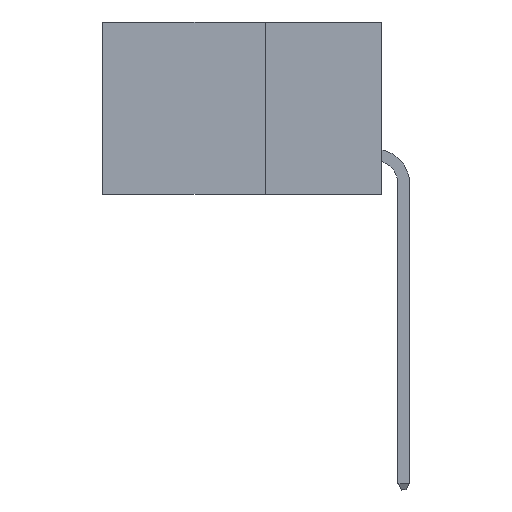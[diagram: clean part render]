
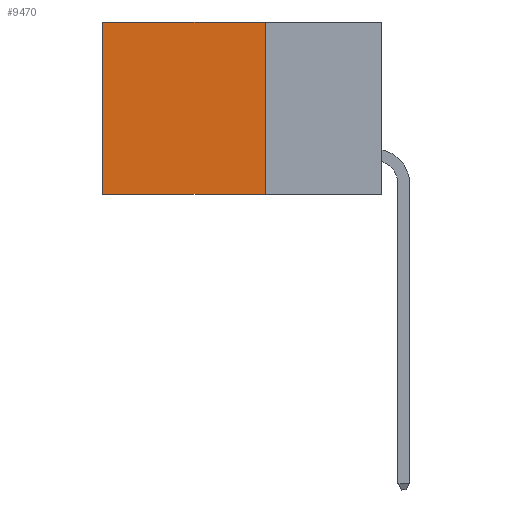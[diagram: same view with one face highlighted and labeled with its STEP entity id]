
A CAD part, left-side view. The second image highlights one B-rep face of the part: STEP entity #9470.
In plain terms, the highlighted planar face has unit normal (-1, 0, 0).
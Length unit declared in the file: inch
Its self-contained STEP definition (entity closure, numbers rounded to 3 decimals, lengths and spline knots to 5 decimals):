
#390 = LINE ( 'NONE', #29003, #17662 ) ;
#4487 = LINE ( 'NONE', #10090, #17136 ) ;
#4966 = VERTEX_POINT ( 'NONE', #17855 ) ;
#5613 = VERTEX_POINT ( 'NONE', #17283 ) ;
#7148 = EDGE_LOOP ( 'NONE', ( #9092, #29058, #9998, #28277 ) ) ;
#8031 = VECTOR ( 'NONE', #18844, 39.37008 ) ;
#8663 = DIRECTION ( 'NONE',  ( 0., 1., 0. ) ) ;
#9092 = ORIENTED_EDGE ( 'NONE', *, *, #27986, .T. ) ;
#9470 = ADVANCED_FACE ( 'NONE', ( #22668 ), #28530, .F. ) ;
#9898 = VECTOR ( 'NONE', #23428, 39.37008 ) ;
#9998 = ORIENTED_EDGE ( 'NONE', *, *, #25482, .F. ) ;
#10090 = CARTESIAN_POINT ( 'NONE',  ( 0.2875, 0.6, 0. ) ) ;
#10237 = VERTEX_POINT ( 'NONE', #28568 ) ;
#12188 = EDGE_CURVE ( 'NONE', #10237, #5613, #390, .T. ) ;
#12823 = DIRECTION ( 'NONE',  ( 1., 0., 0. ) ) ;
#13265 = LINE ( 'NONE', #14539, #8031 ) ;
#13345 = LINE ( 'NONE', #18789, #9898 ) ;
#14539 = CARTESIAN_POINT ( 'NONE',  ( 0.2875, 0.25, 0. ) ) ;
#15705 = AXIS2_PLACEMENT_3D ( 'NONE', #19302, #12823, #17319 ) ;
#17136 = VECTOR ( 'NONE', #25801, 39.37008 ) ;
#17283 = CARTESIAN_POINT ( 'NONE',  ( 0.2875, 0.6, -0.37 ) ) ;
#17319 = DIRECTION ( 'NONE',  ( 0., 0., -1. ) ) ;
#17662 = VECTOR ( 'NONE', #8663, 39.37008 ) ;
#17855 = CARTESIAN_POINT ( 'NONE',  ( 0.2875, 0.6, 0. ) ) ;
#18789 = CARTESIAN_POINT ( 'NONE',  ( 0.2875, 0.25, 0. ) ) ;
#18844 = DIRECTION ( 'NONE',  ( 0., 1., 0. ) ) ;
#19302 = CARTESIAN_POINT ( 'NONE',  ( 0.2875, 0.25, 0. ) ) ;
#22668 = FACE_OUTER_BOUND ( 'NONE', #7148, .T. ) ;
#23428 = DIRECTION ( 'NONE',  ( 0., 0., -1. ) ) ;
#23566 = VERTEX_POINT ( 'NONE', #27305 ) ;
#25482 = EDGE_CURVE ( 'NONE', #23566, #10237, #13345, .T. ) ;
#25801 = DIRECTION ( 'NONE',  ( 0., 0., -1. ) ) ;
#27305 = CARTESIAN_POINT ( 'NONE',  ( 0.2875, 0.25, 0. ) ) ;
#27561 = EDGE_CURVE ( 'NONE', #23566, #4966, #13265, .T. ) ;
#27986 = EDGE_CURVE ( 'NONE', #4966, #5613, #4487, .T. ) ;
#28277 = ORIENTED_EDGE ( 'NONE', *, *, #27561, .T. ) ;
#28530 = PLANE ( 'NONE',  #15705 ) ;
#28568 = CARTESIAN_POINT ( 'NONE',  ( 0.2875, 0.25, -0.37 ) ) ;
#29003 = CARTESIAN_POINT ( 'NONE',  ( 0.2875, 0.25, -0.37 ) ) ;
#29058 = ORIENTED_EDGE ( 'NONE', *, *, #12188, .F. ) ;
